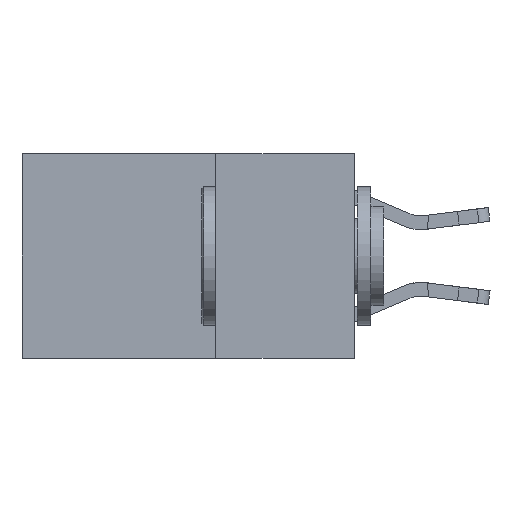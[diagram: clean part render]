
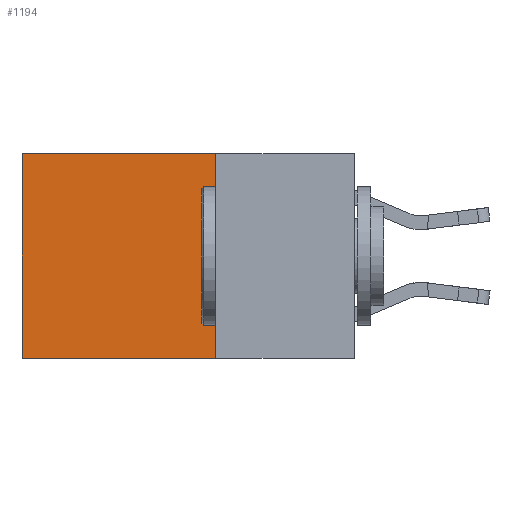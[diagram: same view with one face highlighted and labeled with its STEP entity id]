
A CAD part, left-side view. The second image highlights one B-rep face of the part: STEP entity #1194.
In plain terms, the highlighted planar face has unit normal (-1, 0, 0).
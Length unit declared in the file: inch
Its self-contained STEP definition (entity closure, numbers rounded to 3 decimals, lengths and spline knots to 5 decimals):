
#66 = EDGE_CURVE ( 'NONE', #9608, #26700, #19463, .T. ) ;
#602 = CARTESIAN_POINT ( 'NONE',  ( 0.2625, 0.25, 0. ) ) ;
#1194 = ADVANCED_FACE ( 'NONE', ( #20087 ), #17091, .F. ) ;
#1608 = ORIENTED_EDGE ( 'NONE', *, *, #21423, .T. ) ;
#2779 = ORIENTED_EDGE ( 'NONE', *, *, #19716, .T. ) ;
#3180 = VECTOR ( 'NONE', #3398, 39.37008 ) ;
#3221 = VERTEX_POINT ( 'NONE', #4754 ) ;
#3398 = DIRECTION ( 'NONE',  ( 0., 1., 0. ) ) ;
#3633 = LINE ( 'NONE', #9771, #13603 ) ;
#4426 = CARTESIAN_POINT ( 'NONE',  ( 0.2625, 0.25, 0. ) ) ;
#4754 = CARTESIAN_POINT ( 'NONE',  ( 0.2625, 0.6, 0. ) ) ;
#5154 = ORIENTED_EDGE ( 'NONE', *, *, #19358, .F. ) ;
#6600 = DIRECTION ( 'NONE',  ( 1., 0., 0. ) ) ;
#7155 = EDGE_LOOP ( 'NONE', ( #2779, #5154, #9728, #1608 ) ) ;
#8834 = CARTESIAN_POINT ( 'NONE',  ( 0.2625, 0.6, 0. ) ) ;
#9608 = VERTEX_POINT ( 'NONE', #602 ) ;
#9728 = ORIENTED_EDGE ( 'NONE', *, *, #66, .F. ) ;
#9771 = CARTESIAN_POINT ( 'NONE',  ( 0.2625, 0.25, -0.37 ) ) ;
#10639 = LINE ( 'NONE', #8834, #16244 ) ;
#11647 = DIRECTION ( 'NONE',  ( 0., 0., -1. ) ) ;
#13603 = VECTOR ( 'NONE', #22366, 39.37008 ) ;
#13857 = VECTOR ( 'NONE', #11647, 39.37008 ) ;
#13983 = CARTESIAN_POINT ( 'NONE',  ( 0.2625, 0.25, 0. ) ) ;
#14419 = CARTESIAN_POINT ( 'NONE',  ( 0.2625, 0.25, -0.37 ) ) ;
#14681 = VERTEX_POINT ( 'NONE', #18769 ) ;
#15604 = AXIS2_PLACEMENT_3D ( 'NONE', #4426, #6600, #21314 ) ;
#16244 = VECTOR ( 'NONE', #19318, 39.37008 ) ;
#17091 = PLANE ( 'NONE',  #15604 ) ;
#18769 = CARTESIAN_POINT ( 'NONE',  ( 0.2625, 0.6, -0.37 ) ) ;
#19318 = DIRECTION ( 'NONE',  ( 0., 0., -1. ) ) ;
#19358 = EDGE_CURVE ( 'NONE', #26700, #14681, #3633, .T. ) ;
#19463 = LINE ( 'NONE', #26341, #13857 ) ;
#19716 = EDGE_CURVE ( 'NONE', #3221, #14681, #10639, .T. ) ;
#20059 = LINE ( 'NONE', #13983, #3180 ) ;
#20087 = FACE_OUTER_BOUND ( 'NONE', #7155, .T. ) ;
#21314 = DIRECTION ( 'NONE',  ( 0., 0., -1. ) ) ;
#21423 = EDGE_CURVE ( 'NONE', #9608, #3221, #20059, .T. ) ;
#22366 = DIRECTION ( 'NONE',  ( 0., 1., 0. ) ) ;
#26341 = CARTESIAN_POINT ( 'NONE',  ( 0.2625, 0.25, 0. ) ) ;
#26700 = VERTEX_POINT ( 'NONE', #14419 ) ;
